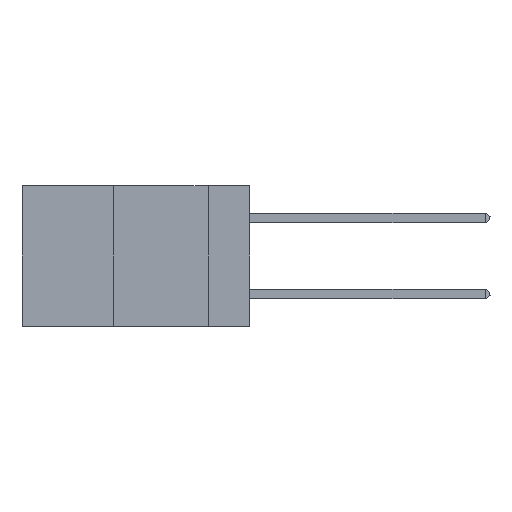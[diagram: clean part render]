
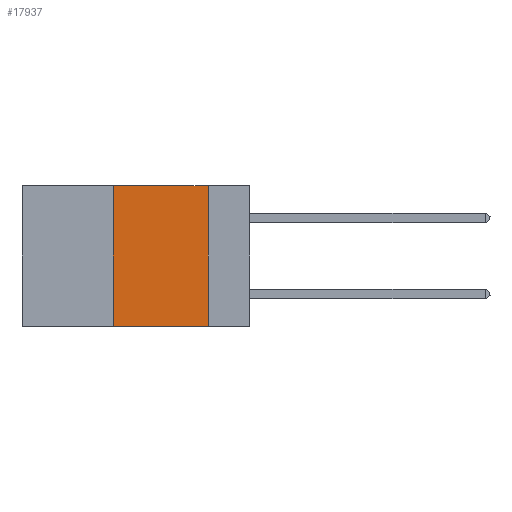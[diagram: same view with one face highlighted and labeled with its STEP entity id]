
A CAD part, left-side view. The second image highlights one B-rep face of the part: STEP entity #17937.
In plain terms, the highlighted planar face has unit normal (-1, 0, 0).
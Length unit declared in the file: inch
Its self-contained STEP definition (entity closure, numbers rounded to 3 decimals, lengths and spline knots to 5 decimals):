
#87 = VERTEX_POINT ( 'NONE', #16643 ) ;
#851 = PLANE ( 'NONE',  #10042 ) ;
#890 = EDGE_CURVE ( 'NONE', #14427, #26110, #26838, .T. ) ;
#3526 = VECTOR ( 'NONE', #13290, 39.37008 ) ;
#5776 = DIRECTION ( 'NONE',  ( 0., 0., -1. ) ) ;
#5909 = EDGE_CURVE ( 'NONE', #13646, #14427, #28450, .T. ) ;
#6180 = VECTOR ( 'NONE', #22207, 39.37008 ) ;
#9456 = LINE ( 'NONE', #10193, #3526 ) ;
#9631 = VECTOR ( 'NONE', #15384, 39.37008 ) ;
#10042 = AXIS2_PLACEMENT_3D ( 'NONE', #10807, #17624, #5776 ) ;
#10193 = CARTESIAN_POINT ( 'NONE',  ( 0., 0.6, -0.37 ) ) ;
#10647 = CARTESIAN_POINT ( 'NONE',  ( 0., 0.36, 0. ) ) ;
#10807 = CARTESIAN_POINT ( 'NONE',  ( 0., 0.6, 0. ) ) ;
#11075 = ORIENTED_EDGE ( 'NONE', *, *, #890, .F. ) ;
#12466 = ORIENTED_EDGE ( 'NONE', *, *, #17178, .T. ) ;
#12534 = CARTESIAN_POINT ( 'NONE',  ( 0., 0.11, 0. ) ) ;
#12800 = CARTESIAN_POINT ( 'NONE',  ( 0., 0.11, -0.37 ) ) ;
#13290 = DIRECTION ( 'NONE',  ( 0., -1., 0. ) ) ;
#13646 = VERTEX_POINT ( 'NONE', #28225 ) ;
#14427 = VERTEX_POINT ( 'NONE', #12534 ) ;
#14919 = CARTESIAN_POINT ( 'NONE',  ( 0., 0.6, 0. ) ) ;
#14948 = EDGE_CURVE ( 'NONE', #87, #13646, #16064, .T. ) ;
#15384 = DIRECTION ( 'NONE',  ( 0., 0., 1. ) ) ;
#16064 = LINE ( 'NONE', #10647, #9631 ) ;
#16456 = ORIENTED_EDGE ( 'NONE', *, *, #14948, .F. ) ;
#16643 = CARTESIAN_POINT ( 'NONE',  ( 0., 0.36, -0.37 ) ) ;
#17178 = EDGE_CURVE ( 'NONE', #87, #26110, #9456, .T. ) ;
#17624 = DIRECTION ( 'NONE',  ( 1., 0., 0. ) ) ;
#17937 = ADVANCED_FACE ( 'NONE', ( #28337 ), #851, .F. ) ;
#18287 = ORIENTED_EDGE ( 'NONE', *, *, #5909, .F. ) ;
#18295 = DIRECTION ( 'NONE',  ( 0., 0., -1. ) ) ;
#20454 = VECTOR ( 'NONE', #18295, 39.37008 ) ;
#22207 = DIRECTION ( 'NONE',  ( 0., -1., 0. ) ) ;
#22645 = EDGE_LOOP ( 'NONE', ( #11075, #18287, #16456, #12466 ) ) ;
#25059 = CARTESIAN_POINT ( 'NONE',  ( 0., 0.11, 0. ) ) ;
#26110 = VERTEX_POINT ( 'NONE', #12800 ) ;
#26838 = LINE ( 'NONE', #25059, #20454 ) ;
#28225 = CARTESIAN_POINT ( 'NONE',  ( 0., 0.36, 0. ) ) ;
#28337 = FACE_OUTER_BOUND ( 'NONE', #22645, .T. ) ;
#28450 = LINE ( 'NONE', #14919, #6180 ) ;
